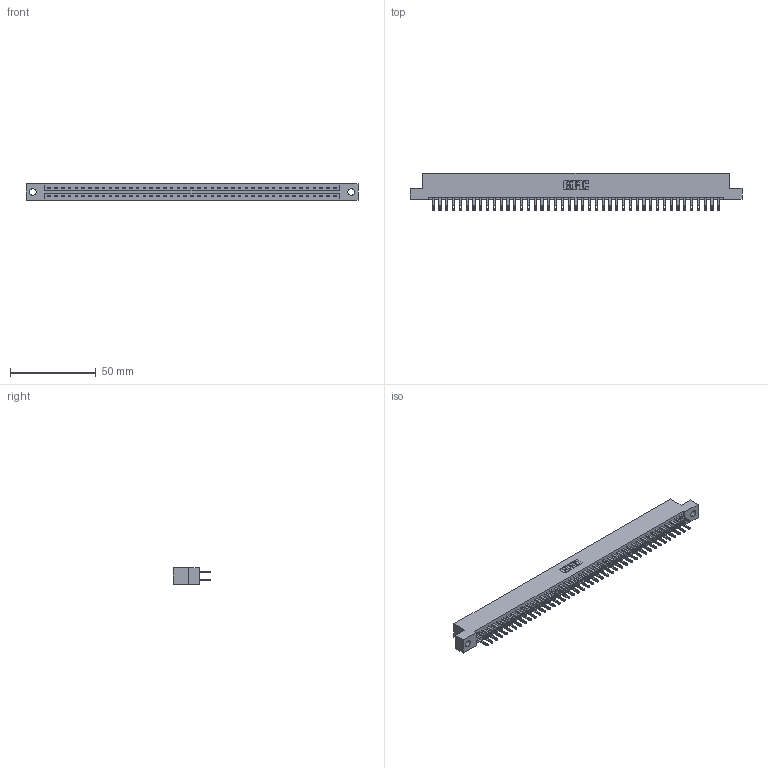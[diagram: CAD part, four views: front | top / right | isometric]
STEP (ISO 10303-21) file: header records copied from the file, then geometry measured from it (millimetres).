
FILE_DESCRIPTION (( 'STEP AP203' ), '1' );
FILE_NAME ('887-086-500-204.STEP', '2020-09-21T05:02:24', ( '' ), ( '' ), 'SwSTEP 2.0', 'SolidWorks 2020', '' );
FILE_SCHEMA (( 'CONFIG_CONTROL_DESIGN' ));
Length unit declared in the file: inch
Products named in the file (3): 345-292-001_345-293-100; 837 Part_Flush Mounting Lugs - 0.156 Dia-TH; 887-086-500-204
Assembly tree (87 placements, depth 2):
  887-086-500-204
    837 Part_Flush Mounting Lugs - 0.156 Dia-TH
    345-292-001_345-293-100  x86
Bounding box: 193.4 x 21.85 x 9.4 mm (x, y, z)
Volume: 20569.8 mm3; surface area: 24015.6 mm2
Topology: 87 solids, 87 shells, 4414 faces, 13469 edges, 8978 vertices
Faces by surface type: plane 2822, cylinder 1592
Entity records: 33143 total; most frequent: CARTESIAN_POINT 5582, ORIENTED_EDGE 5518, DIRECTION 4747, EDGE_CURVE 2759, LINE 2627, VECTOR 2627, VERTEX_POINT 1838, AXIS2_PLACEMENT_3D 1060
